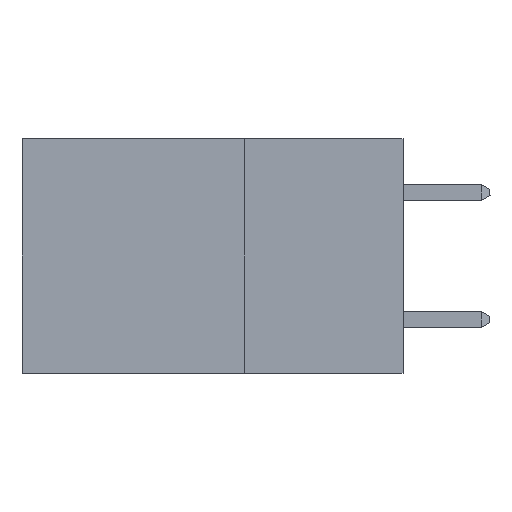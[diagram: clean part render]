
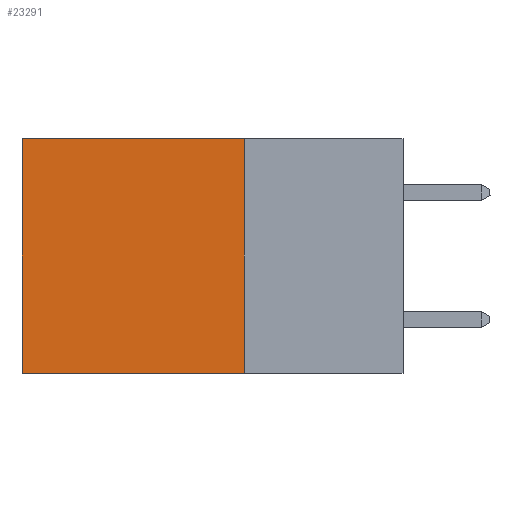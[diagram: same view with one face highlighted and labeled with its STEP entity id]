
A CAD part, left-side view. The second image highlights one B-rep face of the part: STEP entity #23291.
In plain terms, the highlighted planar face has unit normal (-1, 0, 0).
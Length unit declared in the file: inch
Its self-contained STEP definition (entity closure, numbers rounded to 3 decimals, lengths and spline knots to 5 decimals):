
#470 = ORIENTED_EDGE ( 'NONE', *, *, #13284, .T. ) ;
#760 = AXIS2_PLACEMENT_3D ( 'NONE', #27019, #4469, #18070 ) ;
#1117 = VERTEX_POINT ( 'NONE', #25417 ) ;
#1775 = ORIENTED_EDGE ( 'NONE', *, *, #25362, .F. ) ;
#2518 = EDGE_CURVE ( 'NONE', #12714, #14826, #18766, .T. ) ;
#3037 = CARTESIAN_POINT ( 'NONE',  ( 0.2875, 0.25, 0. ) ) ;
#3299 = DIRECTION ( 'NONE',  ( 0., 0., -1. ) ) ;
#4469 = DIRECTION ( 'NONE',  ( 1., 0., 0. ) ) ;
#6057 = LINE ( 'NONE', #3037, #15251 ) ;
#7285 = CARTESIAN_POINT ( 'NONE',  ( 0.2875, 0.25, -0.37 ) ) ;
#7920 = ORIENTED_EDGE ( 'NONE', *, *, #2518, .F. ) ;
#7923 = VECTOR ( 'NONE', #13036, 39.37008 ) ;
#10721 = PLANE ( 'NONE',  #760 ) ;
#11688 = LINE ( 'NONE', #27812, #32339 ) ;
#12500 = CARTESIAN_POINT ( 'NONE',  ( 0.2875, 0.25, 0. ) ) ;
#12658 = DIRECTION ( 'NONE',  ( 0., 1., 0. ) ) ;
#12714 = VERTEX_POINT ( 'NONE', #21349 ) ;
#13036 = DIRECTION ( 'NONE',  ( 0., 0., -1. ) ) ;
#13284 = EDGE_CURVE ( 'NONE', #12714, #1117, #6057, .T. ) ;
#14696 = ORIENTED_EDGE ( 'NONE', *, *, #33377, .T. ) ;
#14826 = VERTEX_POINT ( 'NONE', #18384 ) ;
#15251 = VECTOR ( 'NONE', #30755, 39.37008 ) ;
#15547 = VECTOR ( 'NONE', #12658, 39.37008 ) ;
#18070 = DIRECTION ( 'NONE',  ( 0., 0., -1. ) ) ;
#18384 = CARTESIAN_POINT ( 'NONE',  ( 0.2875, 0.25, -0.37 ) ) ;
#18766 = LINE ( 'NONE', #12500, #7923 ) ;
#21119 = CARTESIAN_POINT ( 'NONE',  ( 0.2875, 0.6, -0.37 ) ) ;
#21349 = CARTESIAN_POINT ( 'NONE',  ( 0.2875, 0.25, 0. ) ) ;
#23291 = ADVANCED_FACE ( 'NONE', ( #29162 ), #10721, .F. ) ;
#23936 = LINE ( 'NONE', #7285, #15547 ) ;
#25362 = EDGE_CURVE ( 'NONE', #14826, #32995, #23936, .T. ) ;
#25417 = CARTESIAN_POINT ( 'NONE',  ( 0.2875, 0.6, 0. ) ) ;
#27019 = CARTESIAN_POINT ( 'NONE',  ( 0.2875, 0.25, 0. ) ) ;
#27812 = CARTESIAN_POINT ( 'NONE',  ( 0.2875, 0.6, 0. ) ) ;
#28943 = EDGE_LOOP ( 'NONE', ( #14696, #1775, #7920, #470 ) ) ;
#29162 = FACE_OUTER_BOUND ( 'NONE', #28943, .T. ) ;
#30755 = DIRECTION ( 'NONE',  ( 0., 1., 0. ) ) ;
#32339 = VECTOR ( 'NONE', #3299, 39.37008 ) ;
#32995 = VERTEX_POINT ( 'NONE', #21119 ) ;
#33377 = EDGE_CURVE ( 'NONE', #1117, #32995, #11688, .T. ) ;
